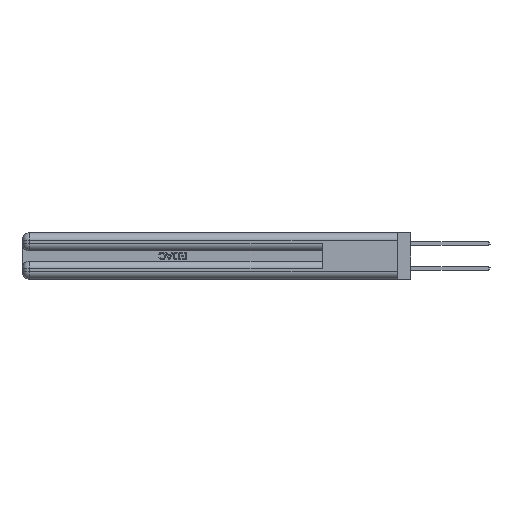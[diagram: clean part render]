
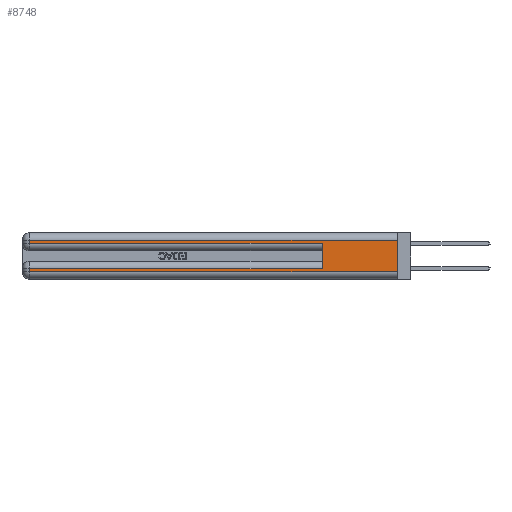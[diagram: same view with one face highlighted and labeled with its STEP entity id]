
A CAD part, left-side view. The second image highlights one B-rep face of the part: STEP entity #8748.
In plain terms, the highlighted planar face has unit normal (-1, 0, 0).
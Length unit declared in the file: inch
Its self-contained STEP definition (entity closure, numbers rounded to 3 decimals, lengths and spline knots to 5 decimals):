
#425 = VERTEX_POINT ( 'NONE', #34270 ) ;
#446 = VECTOR ( 'NONE', #41755, 39.37008 ) ;
#450 = VERTEX_POINT ( 'NONE', #45293 ) ;
#1612 = LINE ( 'NONE', #16135, #446 ) ;
#4409 = LINE ( 'NONE', #35128, #42237 ) ;
#4671 = EDGE_CURVE ( 'NONE', #33751, #19296, #4409, .T. ) ;
#4890 = DIRECTION ( 'NONE',  ( 0., 0., -1. ) ) ;
#5012 = ORIENTED_EDGE ( 'NONE', *, *, #24400, .T. ) ;
#5015 = CARTESIAN_POINT ( 'NONE',  ( 0., 0., 0.06 ) ) ;
#5054 = ORIENTED_EDGE ( 'NONE', *, *, #30563, .T. ) ;
#5260 = LINE ( 'NONE', #43265, #33319 ) ;
#5310 = EDGE_CURVE ( 'NONE', #425, #19292, #45006, .T. ) ;
#6466 = ORIENTED_EDGE ( 'NONE', *, *, #4671, .T. ) ;
#8748 = ADVANCED_FACE ( 'NONE', ( #18335 ), #19402, .F. ) ;
#9500 = LINE ( 'NONE', #19224, #27722 ) ;
#10437 = CARTESIAN_POINT ( 'NONE',  ( 0., 0., 0.085 ) ) ;
#11736 = ORIENTED_EDGE ( 'NONE', *, *, #41712, .T. ) ;
#13208 = DIRECTION ( 'NONE',  ( 0., -1., 0. ) ) ;
#13299 = EDGE_CURVE ( 'NONE', #26011, #19733, #5260, .T. ) ;
#16135 = CARTESIAN_POINT ( 'NONE',  ( 0., 2.94, 0.37 ) ) ;
#17418 = DIRECTION ( 'NONE',  ( 0., -1., 0. ) ) ;
#17643 = AXIS2_PLACEMENT_3D ( 'NONE', #23073, #26760, #4890 ) ;
#17742 = ORIENTED_EDGE ( 'NONE', *, *, #37363, .F. ) ;
#18335 = FACE_OUTER_BOUND ( 'NONE', #35652, .T. ) ;
#19224 = CARTESIAN_POINT ( 'NONE',  ( 0., 0., 0.37 ) ) ;
#19287 = VECTOR ( 'NONE', #17418, 39.37008 ) ;
#19292 = VERTEX_POINT ( 'NONE', #30644 ) ;
#19296 = VERTEX_POINT ( 'NONE', #5015 ) ;
#19402 = PLANE ( 'NONE',  #17643 ) ;
#19733 = VERTEX_POINT ( 'NONE', #29305 ) ;
#22555 = CARTESIAN_POINT ( 'NONE',  ( 0., 0., 0.31 ) ) ;
#22882 = DIRECTION ( 'NONE',  ( 0., 0., -1. ) ) ;
#23073 = CARTESIAN_POINT ( 'NONE',  ( 0., 0., 0.37 ) ) ;
#23219 = VECTOR ( 'NONE', #41032, 39.37008 ) ;
#24400 = EDGE_CURVE ( 'NONE', #19733, #19292, #29073, .T. ) ;
#25138 = DIRECTION ( 'NONE',  ( 0., 0., -1. ) ) ;
#25460 = ORIENTED_EDGE ( 'NONE', *, *, #5310, .F. ) ;
#26011 = VERTEX_POINT ( 'NONE', #34087 ) ;
#26760 = DIRECTION ( 'NONE',  ( 1., 0., 0. ) ) ;
#27042 = VERTEX_POINT ( 'NONE', #32428 ) ;
#27722 = VECTOR ( 'NONE', #22882, 39.37008 ) ;
#29073 = LINE ( 'NONE', #39235, #19287 ) ;
#29305 = CARTESIAN_POINT ( 'NONE',  ( 0., 2.94, 0.285 ) ) ;
#29833 = ORIENTED_EDGE ( 'NONE', *, *, #42940, .T. ) ;
#30563 = EDGE_CURVE ( 'NONE', #425, #27042, #40809, .T. ) ;
#30644 = CARTESIAN_POINT ( 'NONE',  ( 0., 0.6, 0.285 ) ) ;
#31084 = DIRECTION ( 'NONE',  ( 0., 0., 1. ) ) ;
#32428 = CARTESIAN_POINT ( 'NONE',  ( 0., 2.94, 0.085 ) ) ;
#33036 = LINE ( 'NONE', #22555, #23219 ) ;
#33319 = VECTOR ( 'NONE', #25138, 39.37008 ) ;
#33596 = ORIENTED_EDGE ( 'NONE', *, *, #13299, .T. ) ;
#33751 = VERTEX_POINT ( 'NONE', #40545 ) ;
#34087 = CARTESIAN_POINT ( 'NONE',  ( 0., 2.94, 0.31 ) ) ;
#34270 = CARTESIAN_POINT ( 'NONE',  ( 0., 0.6, 0.085 ) ) ;
#35128 = CARTESIAN_POINT ( 'NONE',  ( 0., 0., 0.06 ) ) ;
#35652 = EDGE_LOOP ( 'NONE', ( #17742, #29833, #33596, #5012, #25460, #5054, #11736, #6466 ) ) ;
#35877 = DIRECTION ( 'NONE',  ( 0., 1., 0. ) ) ;
#37363 = EDGE_CURVE ( 'NONE', #450, #19296, #9500, .T. ) ;
#38522 = VECTOR ( 'NONE', #35877, 39.37008 ) ;
#39235 = CARTESIAN_POINT ( 'NONE',  ( 0., 0., 0.285 ) ) ;
#40545 = CARTESIAN_POINT ( 'NONE',  ( 0., 2.94, 0.06 ) ) ;
#40809 = LINE ( 'NONE', #10437, #38522 ) ;
#41032 = DIRECTION ( 'NONE',  ( 0., 1., 0. ) ) ;
#41712 = EDGE_CURVE ( 'NONE', #27042, #33751, #1612, .T. ) ;
#41755 = DIRECTION ( 'NONE',  ( 0., 0., -1. ) ) ;
#42237 = VECTOR ( 'NONE', #13208, 39.37008 ) ;
#42731 = VECTOR ( 'NONE', #31084, 39.37008 ) ;
#42940 = EDGE_CURVE ( 'NONE', #450, #26011, #33036, .T. ) ;
#43265 = CARTESIAN_POINT ( 'NONE',  ( 0., 2.94, 0.37 ) ) ;
#45006 = LINE ( 'NONE', #45599, #42731 ) ;
#45293 = CARTESIAN_POINT ( 'NONE',  ( 0., 0., 0.31 ) ) ;
#45599 = CARTESIAN_POINT ( 'NONE',  ( 0., 0.6, 0.145 ) ) ;
